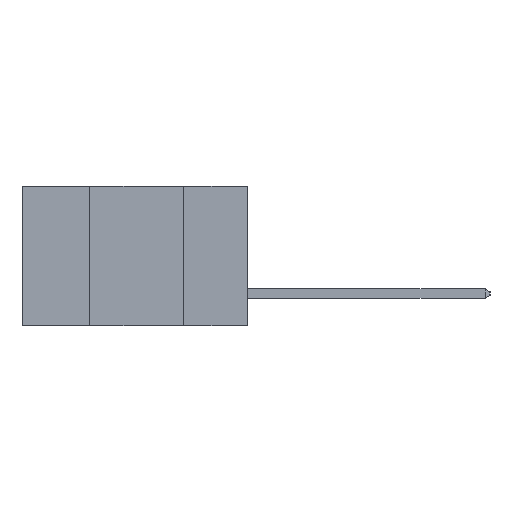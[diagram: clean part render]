
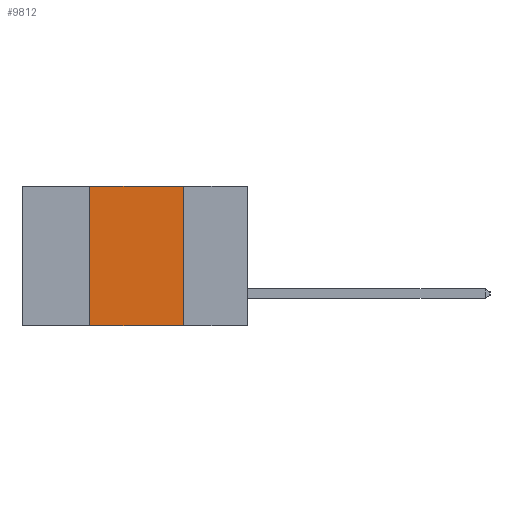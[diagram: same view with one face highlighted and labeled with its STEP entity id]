
A CAD part, left-side view. The second image highlights one B-rep face of the part: STEP entity #9812.
In plain terms, the highlighted planar face has unit normal (-1, 0, 0).
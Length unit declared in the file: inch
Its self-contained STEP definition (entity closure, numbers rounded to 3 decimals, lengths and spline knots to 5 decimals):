
#987 = VERTEX_POINT ( 'NONE', #2063 ) ;
#1060 = AXIS2_PLACEMENT_3D ( 'NONE', #9929, #4366, #14201 ) ;
#2014 = CARTESIAN_POINT ( 'NONE',  ( 0., 0.17, -0.37 ) ) ;
#2063 = CARTESIAN_POINT ( 'NONE',  ( 0., 0.17, 0. ) ) ;
#2156 = ORIENTED_EDGE ( 'NONE', *, *, #6201, .F. ) ;
#2290 = VERTEX_POINT ( 'NONE', #5240 ) ;
#2925 = PLANE ( 'NONE',  #1060 ) ;
#2985 = LINE ( 'NONE', #9523, #17546 ) ;
#4178 = LINE ( 'NONE', #10710, #14516 ) ;
#4312 = EDGE_CURVE ( 'NONE', #2290, #7919, #9445, .T. ) ;
#4366 = DIRECTION ( 'NONE',  ( 1., 0., 0. ) ) ;
#4503 = VERTEX_POINT ( 'NONE', #2014 ) ;
#5240 = CARTESIAN_POINT ( 'NONE',  ( 0., 0.42, -0.37 ) ) ;
#6201 = EDGE_CURVE ( 'NONE', #7919, #987, #2985, .T. ) ;
#6909 = CARTESIAN_POINT ( 'NONE',  ( 0., 0.42, 0. ) ) ;
#7919 = VERTEX_POINT ( 'NONE', #6909 ) ;
#7978 = DIRECTION ( 'NONE',  ( 0., -1., 0. ) ) ;
#8175 = VECTOR ( 'NONE', #13030, 39.37008 ) ;
#9006 = VECTOR ( 'NONE', #17450, 39.37008 ) ;
#9445 = LINE ( 'NONE', #14482, #9006 ) ;
#9523 = CARTESIAN_POINT ( 'NONE',  ( 0., 0.6, 0. ) ) ;
#9812 = ADVANCED_FACE ( 'NONE', ( #16993 ), #2925, .F. ) ;
#9869 = ORIENTED_EDGE ( 'NONE', *, *, #9935, .F. ) ;
#9929 = CARTESIAN_POINT ( 'NONE',  ( 0., 0.6, 0. ) ) ;
#9935 = EDGE_CURVE ( 'NONE', #987, #4503, #11459, .T. ) ;
#10710 = CARTESIAN_POINT ( 'NONE',  ( 0., 0.6, -0.37 ) ) ;
#11459 = LINE ( 'NONE', #11600, #8175 ) ;
#11600 = CARTESIAN_POINT ( 'NONE',  ( 0., 0.17, -0.37 ) ) ;
#12080 = ORIENTED_EDGE ( 'NONE', *, *, #16922, .T. ) ;
#13030 = DIRECTION ( 'NONE',  ( 0., 0., -1. ) ) ;
#13882 = DIRECTION ( 'NONE',  ( 0., -1., 0. ) ) ;
#14201 = DIRECTION ( 'NONE',  ( 0., 0., -1. ) ) ;
#14482 = CARTESIAN_POINT ( 'NONE',  ( 0., 0.42, -0.37 ) ) ;
#14516 = VECTOR ( 'NONE', #7978, 39.37008 ) ;
#16519 = ORIENTED_EDGE ( 'NONE', *, *, #4312, .F. ) ;
#16922 = EDGE_CURVE ( 'NONE', #2290, #4503, #4178, .T. ) ;
#16993 = FACE_OUTER_BOUND ( 'NONE', #18356, .T. ) ;
#17450 = DIRECTION ( 'NONE',  ( 0., 0., 1. ) ) ;
#17546 = VECTOR ( 'NONE', #13882, 39.37008 ) ;
#18356 = EDGE_LOOP ( 'NONE', ( #9869, #2156, #16519, #12080 ) ) ;
